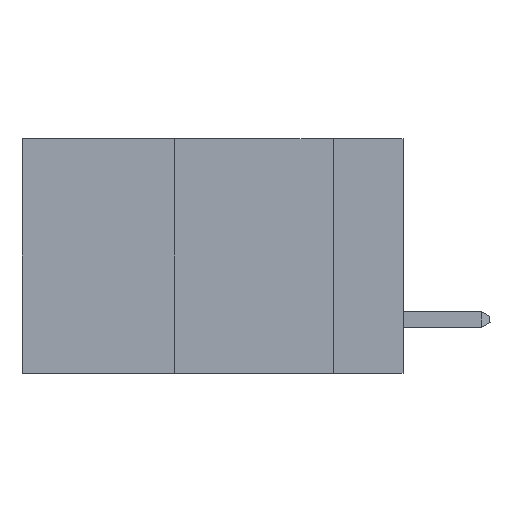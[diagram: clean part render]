
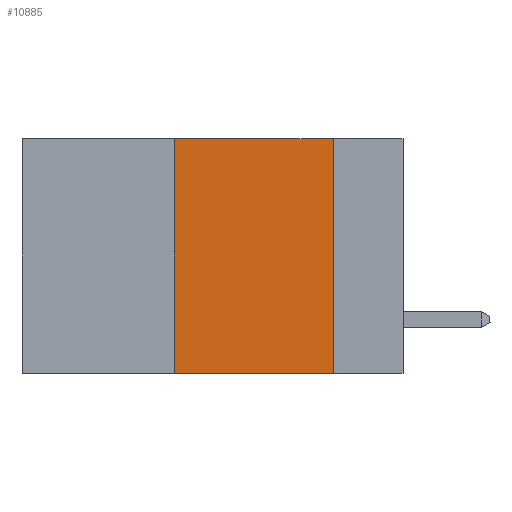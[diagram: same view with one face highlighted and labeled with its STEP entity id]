
A CAD part, left-side view. The second image highlights one B-rep face of the part: STEP entity #10885.
In plain terms, the highlighted planar face has unit normal (-1, 0, 0).
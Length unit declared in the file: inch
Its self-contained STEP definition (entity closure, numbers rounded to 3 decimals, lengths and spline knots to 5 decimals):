
#251 = VECTOR ( 'NONE', #927, 39.37008 ) ;
#572 = CARTESIAN_POINT ( 'NONE',  ( 0., 0.6, -0.37 ) ) ;
#815 = DIRECTION ( 'NONE',  ( 1., 0., 0. ) ) ;
#920 = EDGE_CURVE ( 'NONE', #8219, #10763, #3124, .T. ) ;
#927 = DIRECTION ( 'NONE',  ( 0., 0., 1. ) ) ;
#989 = CARTESIAN_POINT ( 'NONE',  ( 0., 0.11, 0. ) ) ;
#1660 = VECTOR ( 'NONE', #4045, 39.37008 ) ;
#2472 = ORIENTED_EDGE ( 'NONE', *, *, #920, .T. ) ;
#2647 = ORIENTED_EDGE ( 'NONE', *, *, #10890, .F. ) ;
#2961 = CARTESIAN_POINT ( 'NONE',  ( 0., 0.36, 0. ) ) ;
#2979 = CARTESIAN_POINT ( 'NONE',  ( 0., 0.11, -0.37 ) ) ;
#3124 = LINE ( 'NONE', #572, #5467 ) ;
#3415 = CARTESIAN_POINT ( 'NONE',  ( 0., 0.6, 0. ) ) ;
#4033 = EDGE_LOOP ( 'NONE', ( #10449, #6392, #2647, #2472 ) ) ;
#4045 = DIRECTION ( 'NONE',  ( 0., -1., 0. ) ) ;
#5403 = VERTEX_POINT ( 'NONE', #2961 ) ;
#5467 = VECTOR ( 'NONE', #8475, 39.37008 ) ;
#5754 = LINE ( 'NONE', #10830, #1660 ) ;
#5850 = CARTESIAN_POINT ( 'NONE',  ( 0., 0.36, -0.37 ) ) ;
#6392 = ORIENTED_EDGE ( 'NONE', *, *, #9416, .F. ) ;
#6565 = VECTOR ( 'NONE', #6914, 39.37008 ) ;
#6614 = VERTEX_POINT ( 'NONE', #11297 ) ;
#6864 = PLANE ( 'NONE',  #9221 ) ;
#6914 = DIRECTION ( 'NONE',  ( 0., 0., -1. ) ) ;
#7213 = EDGE_CURVE ( 'NONE', #6614, #10763, #11208, .T. ) ;
#8219 = VERTEX_POINT ( 'NONE', #5850 ) ;
#8475 = DIRECTION ( 'NONE',  ( 0., -1., 0. ) ) ;
#8647 = CARTESIAN_POINT ( 'NONE',  ( 0., 0.36, 0. ) ) ;
#9221 = AXIS2_PLACEMENT_3D ( 'NONE', #3415, #815, #9508 ) ;
#9416 = EDGE_CURVE ( 'NONE', #5403, #6614, #5754, .T. ) ;
#9508 = DIRECTION ( 'NONE',  ( 0., 0., -1. ) ) ;
#9574 = LINE ( 'NONE', #8647, #251 ) ;
#9963 = FACE_OUTER_BOUND ( 'NONE', #4033, .T. ) ;
#10449 = ORIENTED_EDGE ( 'NONE', *, *, #7213, .F. ) ;
#10763 = VERTEX_POINT ( 'NONE', #2979 ) ;
#10830 = CARTESIAN_POINT ( 'NONE',  ( 0., 0.6, 0. ) ) ;
#10885 = ADVANCED_FACE ( 'NONE', ( #9963 ), #6864, .F. ) ;
#10890 = EDGE_CURVE ( 'NONE', #8219, #5403, #9574, .T. ) ;
#11208 = LINE ( 'NONE', #989, #6565 ) ;
#11297 = CARTESIAN_POINT ( 'NONE',  ( 0., 0.11, 0. ) ) ;
